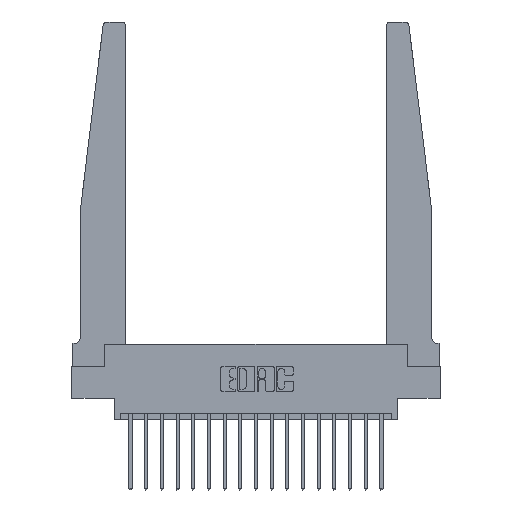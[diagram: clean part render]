
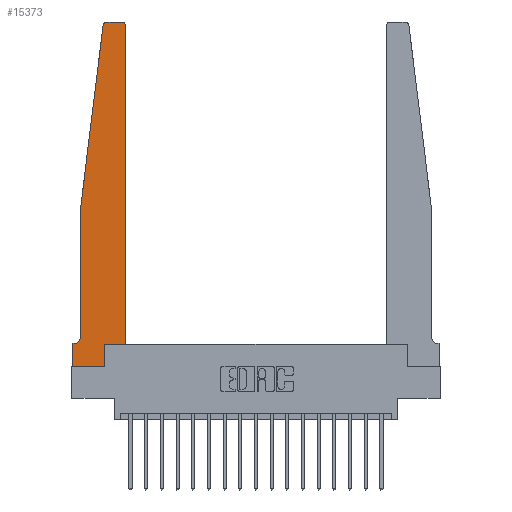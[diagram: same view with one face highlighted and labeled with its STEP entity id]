
A CAD part, top view. The second image highlights one B-rep face of the part: STEP entity #15373.
In plain terms, the highlighted planar face has unit normal (0, 0, 1).
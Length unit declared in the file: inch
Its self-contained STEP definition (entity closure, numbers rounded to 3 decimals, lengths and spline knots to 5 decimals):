
#196 = LINE ( 'NONE', #12436, #17285 ) ;
#235 = VECTOR ( 'NONE', #19605, 39.37008 ) ;
#342 = DIRECTION ( 'NONE',  ( -1., 0., 0. ) ) ;
#390 = ORIENTED_EDGE ( 'NONE', *, *, #8348, .T. ) ;
#448 = CARTESIAN_POINT ( 'NONE',  ( 0.015, 0.1875, 0.37 ) ) ;
#478 = ORIENTED_EDGE ( 'NONE', *, *, #4344, .T. ) ;
#1057 = CARTESIAN_POINT ( 'NONE',  ( 0.2605, 0., 0.37 ) ) ;
#1068 = DIRECTION ( 'NONE',  ( 1., 0., 0. ) ) ;
#1151 = VERTEX_POINT ( 'NONE', #2129 ) ;
#1335 = EDGE_LOOP ( 'NONE', ( #7189, #12999, #478, #13862, #19124, #4171, #9998, #3822, #16275, #2461, #390, #8541 ) ) ;
#1607 = CARTESIAN_POINT ( 'NONE',  ( 0.065, 1.25, 0.37 ) ) ;
#1619 = DIRECTION ( 'NONE',  ( -1., 0., 0. ) ) ;
#1951 = DIRECTION ( 'NONE',  ( 1., 0., 0. ) ) ;
#2129 = CARTESIAN_POINT ( 'NONE',  ( 0.065, 0.2375, 0.37 ) ) ;
#2198 = CARTESIAN_POINT ( 'NONE',  ( 0.065, 1.25, 0.37 ) ) ;
#2251 = VECTOR ( 'NONE', #8397, 39.37008 ) ;
#2305 = VECTOR ( 'NONE', #14725, 39.37008 ) ;
#2418 = DIRECTION ( 'NONE',  ( 0., 0., -1. ) ) ;
#2461 = ORIENTED_EDGE ( 'NONE', *, *, #15745, .T. ) ;
#2627 = VERTEX_POINT ( 'NONE', #4744 ) ;
#2640 = CARTESIAN_POINT ( 'NONE',  ( 0.395, 2.75, 0.37 ) ) ;
#2656 = DIRECTION ( 'NONE',  ( 0., 0., 1. ) ) ;
#2774 = CARTESIAN_POINT ( 'NONE',  ( 0., 0.1875, 0.37 ) ) ;
#3450 = DIRECTION ( 'NONE',  ( 0., -1., 0. ) ) ;
#3822 = ORIENTED_EDGE ( 'NONE', *, *, #7491, .T. ) ;
#3834 = VERTEX_POINT ( 'NONE', #2640 ) ;
#3847 = VECTOR ( 'NONE', #12640, 39.37008 ) ;
#3855 = VECTOR ( 'NONE', #1951, 39.37008 ) ;
#3958 = DIRECTION ( 'NONE',  ( 0., 0., 1. ) ) ;
#4171 = ORIENTED_EDGE ( 'NONE', *, *, #14669, .T. ) ;
#4344 = EDGE_CURVE ( 'NONE', #12507, #7841, #8355, .T. ) ;
#4448 = VERTEX_POINT ( 'NONE', #5716 ) ;
#4684 = CARTESIAN_POINT ( 'NONE',  ( 0., 0., 0.37 ) ) ;
#4744 = CARTESIAN_POINT ( 'NONE',  ( 0.425, 2.72, 0.37 ) ) ;
#4777 = VECTOR ( 'NONE', #3450, 39.37008 ) ;
#4865 = EDGE_CURVE ( 'NONE', #7341, #16705, #9441, .T. ) ;
#4997 = EDGE_CURVE ( 'NONE', #2627, #3834, #17388, .T. ) ;
#5221 = VERTEX_POINT ( 'NONE', #11616 ) ;
#5663 = DIRECTION ( 'NONE',  ( 1., 0., 0. ) ) ;
#5716 = CARTESIAN_POINT ( 'NONE',  ( 0.27653, 2.75, 0.37 ) ) ;
#5759 = CARTESIAN_POINT ( 'NONE',  ( 0.27653, 2.72, 0.37 ) ) ;
#7189 = ORIENTED_EDGE ( 'NONE', *, *, #9671, .T. ) ;
#7341 = VERTEX_POINT ( 'NONE', #1057 ) ;
#7491 = EDGE_CURVE ( 'NONE', #11772, #7341, #11225, .T. ) ;
#7841 = VERTEX_POINT ( 'NONE', #1607 ) ;
#8037 = CARTESIAN_POINT ( 'NONE',  ( 0.2605, 0.18, 0.37 ) ) ;
#8088 = LINE ( 'NONE', #17174, #4777 ) ;
#8140 = DIRECTION ( 'NONE',  ( 1., 0., 0. ) ) ;
#8348 = EDGE_CURVE ( 'NONE', #14690, #2627, #13480, .T. ) ;
#8355 = LINE ( 'NONE', #2198, #2305 ) ;
#8397 = DIRECTION ( 'NONE',  ( -1., 0., 0. ) ) ;
#8510 = VERTEX_POINT ( 'NONE', #448 ) ;
#8541 = ORIENTED_EDGE ( 'NONE', *, *, #4997, .T. ) ;
#8902 = CARTESIAN_POINT ( 'NONE',  ( 0.425, 0.18, 0.37 ) ) ;
#9436 = CARTESIAN_POINT ( 'NONE',  ( 0.425, 0.18, 0.37 ) ) ;
#9441 = LINE ( 'NONE', #8037, #15781 ) ;
#9578 = LINE ( 'NONE', #15662, #3855 ) ;
#9671 = EDGE_CURVE ( 'NONE', #3834, #4448, #9785, .T. ) ;
#9785 = LINE ( 'NONE', #12789, #2251 ) ;
#9794 = EDGE_CURVE ( 'NONE', #4448, #12507, #10309, .T. ) ;
#9998 = ORIENTED_EDGE ( 'NONE', *, *, #15132, .T. ) ;
#10178 = FACE_OUTER_BOUND ( 'NONE', #1335, .T. ) ;
#10309 = CIRCLE ( 'NONE', #17649, 0.03 ) ;
#10590 = AXIS2_PLACEMENT_3D ( 'NONE', #2774, #3958, #1068 ) ;
#10919 = CIRCLE ( 'NONE', #11568, 0.05 ) ;
#11225 = LINE ( 'NONE', #17332, #3847 ) ;
#11568 = AXIS2_PLACEMENT_3D ( 'NONE', #16130, #2418, #342 ) ;
#11616 = CARTESIAN_POINT ( 'NONE',  ( 0., 0.1875, 0.37 ) ) ;
#11772 = VERTEX_POINT ( 'NONE', #15728 ) ;
#12315 = AXIS2_PLACEMENT_3D ( 'NONE', #17321, #18937, #8140 ) ;
#12436 = CARTESIAN_POINT ( 'NONE',  ( 0.065, 0.1875, 0.37 ) ) ;
#12507 = VERTEX_POINT ( 'NONE', #18481 ) ;
#12640 = DIRECTION ( 'NONE',  ( 1., 0., 0. ) ) ;
#12789 = CARTESIAN_POINT ( 'NONE',  ( 0.25, 2.75, 0.37 ) ) ;
#12999 = ORIENTED_EDGE ( 'NONE', *, *, #9794, .T. ) ;
#13382 = PLANE ( 'NONE',  #10590 ) ;
#13480 = LINE ( 'NONE', #8902, #235 ) ;
#13701 = DIRECTION ( 'NONE',  ( 0., -1., 0. ) ) ;
#13793 = EDGE_CURVE ( 'NONE', #7841, #1151, #8088, .T. ) ;
#13862 = ORIENTED_EDGE ( 'NONE', *, *, #13793, .T. ) ;
#14117 = DIRECTION ( 'NONE',  ( 0., 1., 0. ) ) ;
#14669 = EDGE_CURVE ( 'NONE', #8510, #5221, #196, .T. ) ;
#14690 = VERTEX_POINT ( 'NONE', #9436 ) ;
#14725 = DIRECTION ( 'NONE',  ( -0.122, -0.992, 0. ) ) ;
#15132 = EDGE_CURVE ( 'NONE', #5221, #11772, #15209, .T. ) ;
#15192 = CARTESIAN_POINT ( 'NONE',  ( 0.2605, 0.18, 0.37 ) ) ;
#15209 = LINE ( 'NONE', #4684, #16006 ) ;
#15373 = ADVANCED_FACE ( 'NONE', ( #10178 ), #13382, .T. ) ;
#15662 = CARTESIAN_POINT ( 'NONE',  ( 0.425, 0.18, 0.37 ) ) ;
#15728 = CARTESIAN_POINT ( 'NONE',  ( 0., 0., 0.37 ) ) ;
#15745 = EDGE_CURVE ( 'NONE', #16705, #14690, #9578, .T. ) ;
#15781 = VECTOR ( 'NONE', #14117, 39.37008 ) ;
#15876 = EDGE_CURVE ( 'NONE', #1151, #8510, #10919, .T. ) ;
#16006 = VECTOR ( 'NONE', #13701, 39.37008 ) ;
#16130 = CARTESIAN_POINT ( 'NONE',  ( 0.015, 0.2375, 0.37 ) ) ;
#16275 = ORIENTED_EDGE ( 'NONE', *, *, #4865, .T. ) ;
#16705 = VERTEX_POINT ( 'NONE', #15192 ) ;
#17174 = CARTESIAN_POINT ( 'NONE',  ( 0.065, 1.25, 0.37 ) ) ;
#17285 = VECTOR ( 'NONE', #1619, 39.37008 ) ;
#17321 = CARTESIAN_POINT ( 'NONE',  ( 0.395, 2.72, 0.37 ) ) ;
#17332 = CARTESIAN_POINT ( 'NONE',  ( 0., 0., 0.37 ) ) ;
#17388 = CIRCLE ( 'NONE', #12315, 0.03 ) ;
#17649 = AXIS2_PLACEMENT_3D ( 'NONE', #5759, #2656, #5663 ) ;
#18481 = CARTESIAN_POINT ( 'NONE',  ( 0.24675, 2.72367, 0.37 ) ) ;
#18937 = DIRECTION ( 'NONE',  ( 0., 0., 1. ) ) ;
#19124 = ORIENTED_EDGE ( 'NONE', *, *, #15876, .T. ) ;
#19605 = DIRECTION ( 'NONE',  ( 0., 1., 0. ) ) ;
